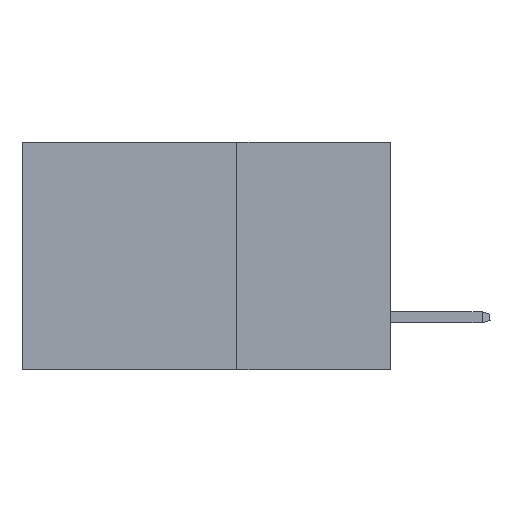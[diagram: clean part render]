
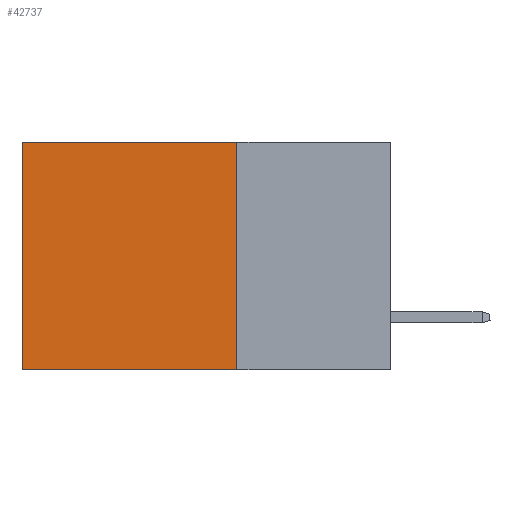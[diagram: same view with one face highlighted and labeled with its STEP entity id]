
A CAD part, left-side view. The second image highlights one B-rep face of the part: STEP entity #42737.
In plain terms, the highlighted planar face has unit normal (-1, 0, 0).
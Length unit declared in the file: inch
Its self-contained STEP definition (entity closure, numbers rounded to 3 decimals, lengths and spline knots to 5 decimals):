
#1819 = DIRECTION ( 'NONE',  ( 0., 1., 0. ) ) ;
#2177 = EDGE_CURVE ( 'NONE', #29137, #16601, #11388, .T. ) ;
#3688 = DIRECTION ( 'NONE',  ( 0., 1., 0. ) ) ;
#4665 = CARTESIAN_POINT ( 'NONE',  ( 0.2875, 0.25, 0. ) ) ;
#5093 = VECTOR ( 'NONE', #1819, 39.37008 ) ;
#5468 = DIRECTION ( 'NONE',  ( 0., 0., -1. ) ) ;
#5512 = EDGE_CURVE ( 'NONE', #43251, #18275, #17904, .T. ) ;
#5633 = AXIS2_PLACEMENT_3D ( 'NONE', #7320, #33146, #32991 ) ;
#6952 = EDGE_CURVE ( 'NONE', #29137, #43251, #35021, .T. ) ;
#7320 = CARTESIAN_POINT ( 'NONE',  ( 0.2875, 0.25, 0. ) ) ;
#10678 = CARTESIAN_POINT ( 'NONE',  ( 0.2875, 0.6, 0. ) ) ;
#11388 = LINE ( 'NONE', #4665, #23974 ) ;
#14820 = CARTESIAN_POINT ( 'NONE',  ( 0.2875, 0.25, 0. ) ) ;
#15485 = DIRECTION ( 'NONE',  ( 0., 0., -1. ) ) ;
#16601 = VERTEX_POINT ( 'NONE', #32149 ) ;
#16658 = LINE ( 'NONE', #45611, #5093 ) ;
#16963 = ORIENTED_EDGE ( 'NONE', *, *, #34796, .F. ) ;
#17904 = LINE ( 'NONE', #20566, #32260 ) ;
#18275 = VERTEX_POINT ( 'NONE', #25320 ) ;
#19776 = ORIENTED_EDGE ( 'NONE', *, *, #6952, .T. ) ;
#19903 = EDGE_LOOP ( 'NONE', ( #24861, #16963, #38311, #19776 ) ) ;
#20566 = CARTESIAN_POINT ( 'NONE',  ( 0.2875, 0.6, 0. ) ) ;
#23974 = VECTOR ( 'NONE', #15485, 39.37008 ) ;
#24861 = ORIENTED_EDGE ( 'NONE', *, *, #5512, .T. ) ;
#25320 = CARTESIAN_POINT ( 'NONE',  ( 0.2875, 0.6, -0.37 ) ) ;
#29137 = VERTEX_POINT ( 'NONE', #42770 ) ;
#29294 = PLANE ( 'NONE',  #5633 ) ;
#29448 = FACE_OUTER_BOUND ( 'NONE', #19903, .T. ) ;
#32149 = CARTESIAN_POINT ( 'NONE',  ( 0.2875, 0.25, -0.37 ) ) ;
#32260 = VECTOR ( 'NONE', #5468, 39.37008 ) ;
#32991 = DIRECTION ( 'NONE',  ( 0., 0., -1. ) ) ;
#33146 = DIRECTION ( 'NONE',  ( 1., 0., 0. ) ) ;
#34796 = EDGE_CURVE ( 'NONE', #16601, #18275, #16658, .T. ) ;
#35021 = LINE ( 'NONE', #14820, #37331 ) ;
#37331 = VECTOR ( 'NONE', #3688, 39.37008 ) ;
#38311 = ORIENTED_EDGE ( 'NONE', *, *, #2177, .F. ) ;
#42737 = ADVANCED_FACE ( 'NONE', ( #29448 ), #29294, .F. ) ;
#42770 = CARTESIAN_POINT ( 'NONE',  ( 0.2875, 0.25, 0. ) ) ;
#43251 = VERTEX_POINT ( 'NONE', #10678 ) ;
#45611 = CARTESIAN_POINT ( 'NONE',  ( 0.2875, 0.25, -0.37 ) ) ;
